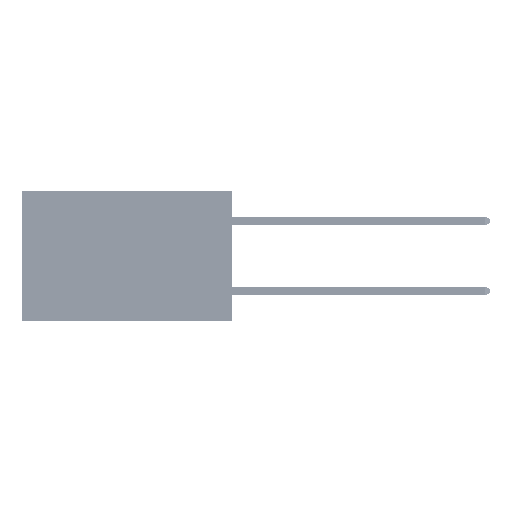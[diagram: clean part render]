
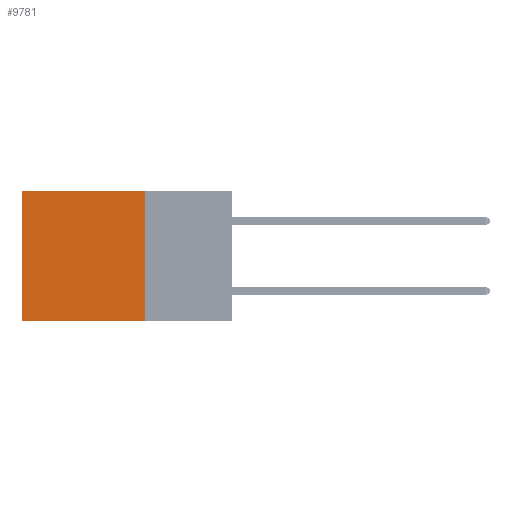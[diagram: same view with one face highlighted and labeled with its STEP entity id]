
A CAD part, left-side view. The second image highlights one B-rep face of the part: STEP entity #9781.
In plain terms, the highlighted planar face has unit normal (-1, 0, 0).
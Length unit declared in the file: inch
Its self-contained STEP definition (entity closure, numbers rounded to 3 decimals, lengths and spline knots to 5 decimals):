
#542 = VERTEX_POINT ( 'NONE', #18968 ) ;
#1723 = ORIENTED_EDGE ( 'NONE', *, *, #5987, .F. ) ;
#2907 = LINE ( 'NONE', #15740, #50780 ) ;
#5987 = EDGE_CURVE ( 'NONE', #36757, #542, #17854, .T. ) ;
#8097 = CARTESIAN_POINT ( 'NONE',  ( 0.2875, 0.25, 0. ) ) ;
#9781 = ADVANCED_FACE ( 'NONE', ( #19864 ), #32627, .F. ) ;
#11233 = AXIS2_PLACEMENT_3D ( 'NONE', #8097, #12388, #28622 ) ;
#12388 = DIRECTION ( 'NONE',  ( 1., 0., 0. ) ) ;
#14113 = CARTESIAN_POINT ( 'NONE',  ( 0.2875, 0.25, -0.37 ) ) ;
#14829 = EDGE_LOOP ( 'NONE', ( #33465, #1723, #25283, #39107 ) ) ;
#14995 = CARTESIAN_POINT ( 'NONE',  ( 0.2875, 0.6, 0. ) ) ;
#15740 = CARTESIAN_POINT ( 'NONE',  ( 0.2875, 0.25, 0. ) ) ;
#17854 = LINE ( 'NONE', #14113, #27701 ) ;
#18653 = CARTESIAN_POINT ( 'NONE',  ( 0.2875, 0.25, -0.37 ) ) ;
#18968 = CARTESIAN_POINT ( 'NONE',  ( 0.2875, 0.6, -0.37 ) ) ;
#19206 = DIRECTION ( 'NONE',  ( 0., 0., -1. ) ) ;
#19864 = FACE_OUTER_BOUND ( 'NONE', #14829, .T. ) ;
#23784 = DIRECTION ( 'NONE',  ( 0., 0., -1. ) ) ;
#23864 = EDGE_CURVE ( 'NONE', #42471, #542, #51542, .T. ) ;
#25283 = ORIENTED_EDGE ( 'NONE', *, *, #34157, .F. ) ;
#26805 = EDGE_CURVE ( 'NONE', #27441, #42471, #2907, .T. ) ;
#27441 = VERTEX_POINT ( 'NONE', #38966 ) ;
#27701 = VECTOR ( 'NONE', #50411, 39.37008 ) ;
#27715 = LINE ( 'NONE', #35459, #32793 ) ;
#28622 = DIRECTION ( 'NONE',  ( 0., 0., -1. ) ) ;
#32627 = PLANE ( 'NONE',  #11233 ) ;
#32793 = VECTOR ( 'NONE', #19206, 39.37008 ) ;
#33465 = ORIENTED_EDGE ( 'NONE', *, *, #23864, .T. ) ;
#34157 = EDGE_CURVE ( 'NONE', #27441, #36757, #27715, .T. ) ;
#35459 = CARTESIAN_POINT ( 'NONE',  ( 0.2875, 0.25, 0. ) ) ;
#36517 = CARTESIAN_POINT ( 'NONE',  ( 0.2875, 0.6, 0. ) ) ;
#36757 = VERTEX_POINT ( 'NONE', #18653 ) ;
#36915 = VECTOR ( 'NONE', #23784, 39.37008 ) ;
#38966 = CARTESIAN_POINT ( 'NONE',  ( 0.2875, 0.25, 0. ) ) ;
#39107 = ORIENTED_EDGE ( 'NONE', *, *, #26805, .T. ) ;
#42471 = VERTEX_POINT ( 'NONE', #36517 ) ;
#47745 = DIRECTION ( 'NONE',  ( 0., 1., 0. ) ) ;
#50411 = DIRECTION ( 'NONE',  ( 0., 1., 0. ) ) ;
#50780 = VECTOR ( 'NONE', #47745, 39.37008 ) ;
#51542 = LINE ( 'NONE', #14995, #36915 ) ;
